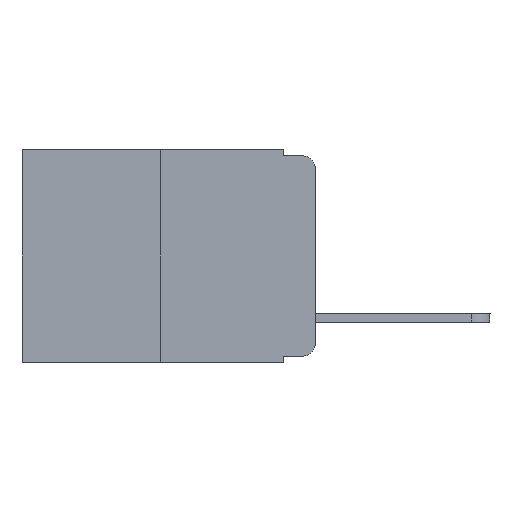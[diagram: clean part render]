
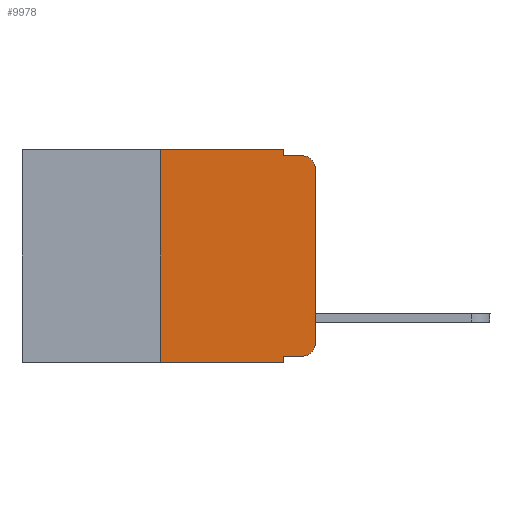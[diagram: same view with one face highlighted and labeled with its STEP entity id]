
A CAD part, left-side view. The second image highlights one B-rep face of the part: STEP entity #9978.
In plain terms, the highlighted planar face has unit normal (-1, 0, 0).
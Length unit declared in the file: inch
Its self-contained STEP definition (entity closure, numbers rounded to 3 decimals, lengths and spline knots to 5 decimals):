
#182 = AXIS2_PLACEMENT_3D ( 'NONE', #4360, #1828, #7399 ) ;
#438 = ORIENTED_EDGE ( 'NONE', *, *, #12536, .F. ) ;
#567 = VECTOR ( 'NONE', #17670, 39.37008 ) ;
#694 = LINE ( 'NONE', #13192, #10860 ) ;
#1359 = VECTOR ( 'NONE', #10033, 39.37008 ) ;
#1576 = VERTEX_POINT ( 'NONE', #8285 ) ;
#1724 = ORIENTED_EDGE ( 'NONE', *, *, #4023, .T. ) ;
#1810 = DIRECTION ( 'NONE',  ( 0., 0., 1. ) ) ;
#1828 = DIRECTION ( 'NONE',  ( -1., 0., 0. ) ) ;
#2139 = ORIENTED_EDGE ( 'NONE', *, *, #4222, .T. ) ;
#2652 = LINE ( 'NONE', #5568, #11111 ) ;
#3104 = EDGE_CURVE ( 'NONE', #1576, #3733, #2652, .T. ) ;
#3187 = DIRECTION ( 'NONE',  ( 0., -1., 0. ) ) ;
#3271 = EDGE_CURVE ( 'NONE', #3651, #5821, #12095, .T. ) ;
#3395 = DIRECTION ( 'NONE',  ( 0., 0., -1. ) ) ;
#3551 = VERTEX_POINT ( 'NONE', #9988 ) ;
#3651 = VERTEX_POINT ( 'NONE', #4783 ) ;
#3690 = CIRCLE ( 'NONE', #12715, 0.02 ) ;
#3733 = VERTEX_POINT ( 'NONE', #17653 ) ;
#3764 = ORIENTED_EDGE ( 'NONE', *, *, #12693, .F. ) ;
#3853 = VECTOR ( 'NONE', #17626, 39.37008 ) ;
#4023 = EDGE_CURVE ( 'NONE', #17996, #1576, #3690, .T. ) ;
#4222 = EDGE_CURVE ( 'NONE', #3733, #13606, #17984, .T. ) ;
#4360 = CARTESIAN_POINT ( 'NONE',  ( 0., 0.02, -0.03 ) ) ;
#4367 = EDGE_CURVE ( 'NONE', #16985, #17996, #11394, .T. ) ;
#4594 = CARTESIAN_POINT ( 'NONE',  ( 0., 0.051, -0.333 ) ) ;
#4783 = CARTESIAN_POINT ( 'NONE',  ( 0., 0.25, -0.343 ) ) ;
#5562 = DIRECTION ( 'NONE',  ( 0., 0., 1. ) ) ;
#5568 = CARTESIAN_POINT ( 'NONE',  ( 0., 0., 0. ) ) ;
#5742 = ORIENTED_EDGE ( 'NONE', *, *, #3271, .T. ) ;
#5821 = VERTEX_POINT ( 'NONE', #17693 ) ;
#7123 = CARTESIAN_POINT ( 'NONE',  ( 0., 0.051, -0.01 ) ) ;
#7399 = DIRECTION ( 'NONE',  ( 0., 0., -1. ) ) ;
#7863 = VERTEX_POINT ( 'NONE', #17568 ) ;
#8193 = CARTESIAN_POINT ( 'NONE',  ( 0., 0.051, -0.01 ) ) ;
#8285 = CARTESIAN_POINT ( 'NONE',  ( 0., 0., -0.313 ) ) ;
#8578 = LINE ( 'NONE', #7123, #9101 ) ;
#8778 = DIRECTION ( 'NONE',  ( -1., 0., 0. ) ) ;
#8810 = VECTOR ( 'NONE', #5562, 39.37008 ) ;
#9101 = VECTOR ( 'NONE', #3187, 39.37008 ) ;
#9665 = CARTESIAN_POINT ( 'NONE',  ( 0., 0.051, 0. ) ) ;
#9749 = ORIENTED_EDGE ( 'NONE', *, *, #3104, .T. ) ;
#9978 = ADVANCED_FACE ( 'NONE', ( #14399 ), #10192, .F. ) ;
#9988 = CARTESIAN_POINT ( 'NONE',  ( 0., 0.25, 0. ) ) ;
#10033 = DIRECTION ( 'NONE',  ( 0., -1., 0. ) ) ;
#10192 = PLANE ( 'NONE',  #14893 ) ;
#10385 = LINE ( 'NONE', #11761, #13762 ) ;
#10793 = ORIENTED_EDGE ( 'NONE', *, *, #16643, .F. ) ;
#10860 = VECTOR ( 'NONE', #12823, 39.37008 ) ;
#11024 = LINE ( 'NONE', #9665, #3853 ) ;
#11111 = VECTOR ( 'NONE', #1810, 39.37008 ) ;
#11394 = LINE ( 'NONE', #16982, #1359 ) ;
#11596 = CARTESIAN_POINT ( 'NONE',  ( 0., 0.02, -0.01 ) ) ;
#11652 = DIRECTION ( 'NONE',  ( 1., 0., 0. ) ) ;
#11761 = CARTESIAN_POINT ( 'NONE',  ( 0., 0.473, 0. ) ) ;
#11883 = ORIENTED_EDGE ( 'NONE', *, *, #4367, .T. ) ;
#12095 = LINE ( 'NONE', #15848, #567 ) ;
#12536 = EDGE_CURVE ( 'NONE', #7863, #16482, #11024, .T. ) ;
#12693 = EDGE_CURVE ( 'NONE', #3651, #3551, #15496, .T. ) ;
#12715 = AXIS2_PLACEMENT_3D ( 'NONE', #14435, #8778, #3395 ) ;
#12823 = DIRECTION ( 'NONE',  ( 0., 0., -1. ) ) ;
#12835 = EDGE_CURVE ( 'NONE', #3551, #7863, #10385, .T. ) ;
#12990 = ORIENTED_EDGE ( 'NONE', *, *, #17944, .F. ) ;
#13192 = CARTESIAN_POINT ( 'NONE',  ( 0., 0.051, 0. ) ) ;
#13606 = VERTEX_POINT ( 'NONE', #11596 ) ;
#13762 = VECTOR ( 'NONE', #14587, 39.37008 ) ;
#13954 = CARTESIAN_POINT ( 'NONE',  ( 0., 0.25, 0. ) ) ;
#14399 = FACE_OUTER_BOUND ( 'NONE', #15276, .T. ) ;
#14435 = CARTESIAN_POINT ( 'NONE',  ( 0., 0.02, -0.313 ) ) ;
#14587 = DIRECTION ( 'NONE',  ( 0., -1., 0. ) ) ;
#14893 = AXIS2_PLACEMENT_3D ( 'NONE', #15762, #11652, #17239 ) ;
#15276 = EDGE_LOOP ( 'NONE', ( #9749, #2139, #12990, #438, #16516, #3764, #5742, #10793, #11883, #1724 ) ) ;
#15496 = LINE ( 'NONE', #13954, #8810 ) ;
#15762 = CARTESIAN_POINT ( 'NONE',  ( 0., 0.473, 0. ) ) ;
#15848 = CARTESIAN_POINT ( 'NONE',  ( 0., 0.473, -0.343 ) ) ;
#16054 = CARTESIAN_POINT ( 'NONE',  ( 0., 0.02, -0.333 ) ) ;
#16482 = VERTEX_POINT ( 'NONE', #8193 ) ;
#16516 = ORIENTED_EDGE ( 'NONE', *, *, #12835, .F. ) ;
#16643 = EDGE_CURVE ( 'NONE', #16985, #5821, #694, .T. ) ;
#16982 = CARTESIAN_POINT ( 'NONE',  ( 0., 0.051, -0.333 ) ) ;
#16985 = VERTEX_POINT ( 'NONE', #4594 ) ;
#17239 = DIRECTION ( 'NONE',  ( 0., 0., -1. ) ) ;
#17568 = CARTESIAN_POINT ( 'NONE',  ( 0., 0.051, 0. ) ) ;
#17626 = DIRECTION ( 'NONE',  ( 0., 0., -1. ) ) ;
#17653 = CARTESIAN_POINT ( 'NONE',  ( 0., 0., -0.03 ) ) ;
#17670 = DIRECTION ( 'NONE',  ( 0., -1., 0. ) ) ;
#17693 = CARTESIAN_POINT ( 'NONE',  ( 0., 0.051, -0.343 ) ) ;
#17944 = EDGE_CURVE ( 'NONE', #16482, #13606, #8578, .T. ) ;
#17984 = CIRCLE ( 'NONE', #182, 0.02 ) ;
#17996 = VERTEX_POINT ( 'NONE', #16054 ) ;
